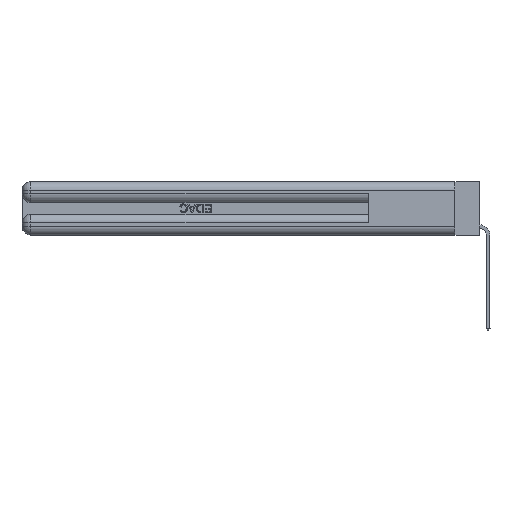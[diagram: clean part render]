
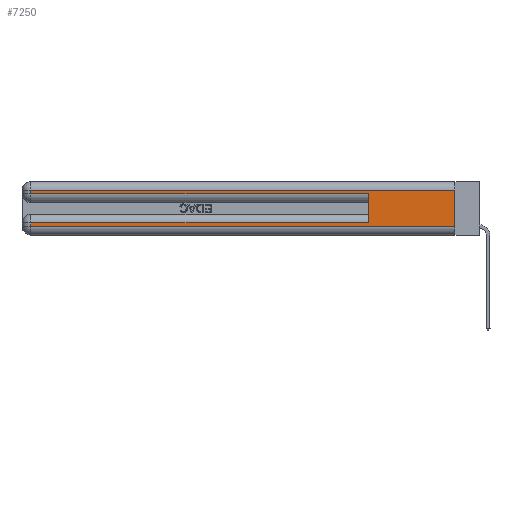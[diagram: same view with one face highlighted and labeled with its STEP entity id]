
A CAD part, left-side view. The second image highlights one B-rep face of the part: STEP entity #7250.
In plain terms, the highlighted planar face has unit normal (-1, 0, 0).
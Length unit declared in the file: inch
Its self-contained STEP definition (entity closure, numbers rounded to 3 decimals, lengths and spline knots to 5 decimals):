
#9 = LINE ( 'NONE', #26282, #449 ) ;
#321 = CARTESIAN_POINT ( 'NONE',  ( 0., 0., 0.31 ) ) ;
#449 = VECTOR ( 'NONE', #6211, 39.37008 ) ;
#1626 = AXIS2_PLACEMENT_3D ( 'NONE', #9234, #2318, #24897 ) ;
#2318 = DIRECTION ( 'NONE',  ( 1., 0., 0. ) ) ;
#2408 = CARTESIAN_POINT ( 'NONE',  ( 0., 0., 0.06 ) ) ;
#2726 = VERTEX_POINT ( 'NONE', #25260 ) ;
#4716 = CARTESIAN_POINT ( 'NONE',  ( 0., 0.6, 0.285 ) ) ;
#4820 = ORIENTED_EDGE ( 'NONE', *, *, #16015, .T. ) ;
#4990 = ORIENTED_EDGE ( 'NONE', *, *, #15650, .T. ) ;
#5286 = VERTEX_POINT ( 'NONE', #12943 ) ;
#5499 = CARTESIAN_POINT ( 'NONE',  ( 0., 2.94, 0.085 ) ) ;
#5675 = VECTOR ( 'NONE', #28348, 39.37008 ) ;
#6211 = DIRECTION ( 'NONE',  ( 0., -1., 0. ) ) ;
#6361 = CARTESIAN_POINT ( 'NONE',  ( 0., 2.94, 0.31 ) ) ;
#6817 = ORIENTED_EDGE ( 'NONE', *, *, #23149, .F. ) ;
#7090 = EDGE_CURVE ( 'NONE', #14026, #11927, #13031, .T. ) ;
#7192 = LINE ( 'NONE', #10258, #15088 ) ;
#7250 = ADVANCED_FACE ( 'NONE', ( #13477 ), #22433, .F. ) ;
#8361 = CARTESIAN_POINT ( 'NONE',  ( 0., 0., 0.285 ) ) ;
#9003 = VECTOR ( 'NONE', #25333, 39.37008 ) ;
#9234 = CARTESIAN_POINT ( 'NONE',  ( 0., 0., 0.37 ) ) ;
#9636 = LINE ( 'NONE', #16662, #17587 ) ;
#10001 = ORIENTED_EDGE ( 'NONE', *, *, #17137, .T. ) ;
#10137 = EDGE_LOOP ( 'NONE', ( #25611, #23223, #4990, #13929, #6817, #4820, #10001, #14505 ) ) ;
#10258 = CARTESIAN_POINT ( 'NONE',  ( 0., 0.6, 0.145 ) ) ;
#11927 = VERTEX_POINT ( 'NONE', #4716 ) ;
#12943 = CARTESIAN_POINT ( 'NONE',  ( 0., 2.94, 0.06 ) ) ;
#13031 = LINE ( 'NONE', #8361, #14182 ) ;
#13477 = FACE_OUTER_BOUND ( 'NONE', #10137, .T. ) ;
#13929 = ORIENTED_EDGE ( 'NONE', *, *, #7090, .T. ) ;
#14026 = VERTEX_POINT ( 'NONE', #16459 ) ;
#14158 = DIRECTION ( 'NONE',  ( 0., 0., -1. ) ) ;
#14182 = VECTOR ( 'NONE', #19790, 39.37008 ) ;
#14505 = ORIENTED_EDGE ( 'NONE', *, *, #25267, .T. ) ;
#15088 = VECTOR ( 'NONE', #16872, 39.37008 ) ;
#15650 = EDGE_CURVE ( 'NONE', #20513, #14026, #27109, .T. ) ;
#16015 = EDGE_CURVE ( 'NONE', #2726, #19533, #18160, .T. ) ;
#16091 = VECTOR ( 'NONE', #27693, 39.37008 ) ;
#16459 = CARTESIAN_POINT ( 'NONE',  ( 0., 2.94, 0.285 ) ) ;
#16537 = CARTESIAN_POINT ( 'NONE',  ( 0., 0., 0.085 ) ) ;
#16662 = CARTESIAN_POINT ( 'NONE',  ( 0., 2.94, 0.37 ) ) ;
#16872 = DIRECTION ( 'NONE',  ( 0., 0., 1. ) ) ;
#16925 = VECTOR ( 'NONE', #18683, 39.37008 ) ;
#17137 = EDGE_CURVE ( 'NONE', #19533, #5286, #9636, .T. ) ;
#17259 = VERTEX_POINT ( 'NONE', #321 ) ;
#17587 = VECTOR ( 'NONE', #14158, 39.37008 ) ;
#18160 = LINE ( 'NONE', #16537, #9003 ) ;
#18683 = DIRECTION ( 'NONE',  ( 0., 0., -1. ) ) ;
#19408 = LINE ( 'NONE', #21768, #5675 ) ;
#19533 = VERTEX_POINT ( 'NONE', #5499 ) ;
#19790 = DIRECTION ( 'NONE',  ( 0., -1., 0. ) ) ;
#20513 = VERTEX_POINT ( 'NONE', #6361 ) ;
#20538 = CARTESIAN_POINT ( 'NONE',  ( 0., 2.94, 0.37 ) ) ;
#21156 = EDGE_CURVE ( 'NONE', #17259, #20513, #19408, .T. ) ;
#21297 = CARTESIAN_POINT ( 'NONE',  ( 0., 0., 0.37 ) ) ;
#21763 = VERTEX_POINT ( 'NONE', #2408 ) ;
#21768 = CARTESIAN_POINT ( 'NONE',  ( 0., 0., 0.31 ) ) ;
#22433 = PLANE ( 'NONE',  #1626 ) ;
#23149 = EDGE_CURVE ( 'NONE', #2726, #11927, #7192, .T. ) ;
#23223 = ORIENTED_EDGE ( 'NONE', *, *, #21156, .T. ) ;
#24897 = DIRECTION ( 'NONE',  ( 0., 0., -1. ) ) ;
#25260 = CARTESIAN_POINT ( 'NONE',  ( 0., 0.6, 0.085 ) ) ;
#25267 = EDGE_CURVE ( 'NONE', #5286, #21763, #9, .T. ) ;
#25333 = DIRECTION ( 'NONE',  ( 0., 1., 0. ) ) ;
#25611 = ORIENTED_EDGE ( 'NONE', *, *, #26250, .F. ) ;
#25711 = LINE ( 'NONE', #21297, #16925 ) ;
#26250 = EDGE_CURVE ( 'NONE', #17259, #21763, #25711, .T. ) ;
#26282 = CARTESIAN_POINT ( 'NONE',  ( 0., 0., 0.06 ) ) ;
#27109 = LINE ( 'NONE', #20538, #16091 ) ;
#27693 = DIRECTION ( 'NONE',  ( 0., 0., -1. ) ) ;
#28348 = DIRECTION ( 'NONE',  ( 0., 1., 0. ) ) ;
